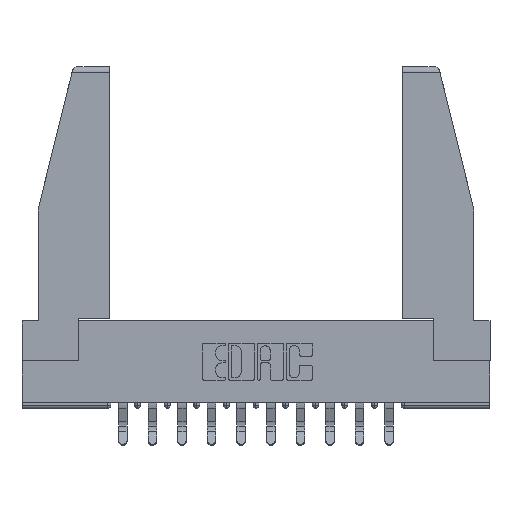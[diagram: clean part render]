
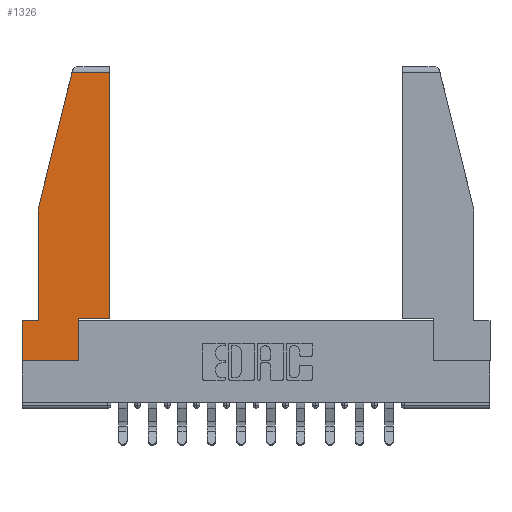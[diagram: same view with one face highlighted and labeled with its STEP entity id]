
A CAD part, top view. The second image highlights one B-rep face of the part: STEP entity #1326.
In plain terms, the highlighted planar face has unit normal (0, 0, 1).
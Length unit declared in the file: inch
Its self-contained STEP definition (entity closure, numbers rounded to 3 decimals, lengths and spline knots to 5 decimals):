
#252 = VERTEX_POINT ( 'NONE', #12248 ) ;
#356 = DIRECTION ( 'NONE',  ( 0., -1., 0. ) ) ;
#734 = VECTOR ( 'NONE', #16196, 39.37008 ) ;
#753 = EDGE_CURVE ( 'NONE', #14464, #252, #7016, .T. ) ;
#931 = LINE ( 'NONE', #16263, #734 ) ;
#1299 = DIRECTION ( 'NONE',  ( -1., 0., 0. ) ) ;
#1326 = ADVANCED_FACE ( 'NONE', ( #11200 ), #15914, .T. ) ;
#1522 = LINE ( 'NONE', #8565, #10340 ) ;
#1701 = ORIENTED_EDGE ( 'NONE', *, *, #16197, .T. ) ;
#1985 = CARTESIAN_POINT ( 'NONE',  ( 0., 0.21, 0. ) ) ;
#2425 = DIRECTION ( 'NONE',  ( 0., -1., 0. ) ) ;
#3075 = EDGE_CURVE ( 'NONE', #12537, #5365, #11976, .T. ) ;
#3438 = VECTOR ( 'NONE', #1299, 39.37008 ) ;
#3572 = AXIS2_PLACEMENT_3D ( 'NONE', #12133, #5305, #13537 ) ;
#3636 = ORIENTED_EDGE ( 'NONE', *, *, #753, .T. ) ;
#3857 = CARTESIAN_POINT ( 'NONE',  ( 0., 1.52, 0. ) ) ;
#3923 = LINE ( 'NONE', #7523, #7714 ) ;
#4190 = VECTOR ( 'NONE', #8435, 39.37008 ) ;
#4196 = DIRECTION ( 'NONE',  ( -0.239, -0.971, 0. ) ) ;
#4378 = CARTESIAN_POINT ( 'NONE',  ( 0., 0., 0. ) ) ;
#4579 = EDGE_CURVE ( 'NONE', #252, #11981, #16111, .T. ) ;
#4947 = EDGE_CURVE ( 'NONE', #11981, #9385, #11437, .T. ) ;
#5299 = VECTOR ( 'NONE', #14900, 39.37008 ) ;
#5305 = DIRECTION ( 'NONE',  ( 0., 0., 1. ) ) ;
#5344 = CARTESIAN_POINT ( 'NONE',  ( 0.297, 0., 0. ) ) ;
#5365 = VERTEX_POINT ( 'NONE', #10598 ) ;
#5548 = ORIENTED_EDGE ( 'NONE', *, *, #4947, .T. ) ;
#5598 = CARTESIAN_POINT ( 'NONE',  ( 0.297, 0.223, 0. ) ) ;
#5973 = VECTOR ( 'NONE', #4196, 39.37008 ) ;
#6244 = VERTEX_POINT ( 'NONE', #1985 ) ;
#6564 = CARTESIAN_POINT ( 'NONE',  ( 0.297, 0.223, 0. ) ) ;
#6566 = LINE ( 'NONE', #6564, #5299 ) ;
#6943 = ORIENTED_EDGE ( 'NONE', *, *, #4579, .T. ) ;
#7007 = ORIENTED_EDGE ( 'NONE', *, *, #16994, .T. ) ;
#7016 = LINE ( 'NONE', #3857, #3438 ) ;
#7520 = CARTESIAN_POINT ( 'NONE',  ( 0., 0., 0. ) ) ;
#7523 = CARTESIAN_POINT ( 'NONE',  ( 0.461, 0.223, 0. ) ) ;
#7702 = EDGE_CURVE ( 'NONE', #5365, #8466, #13246, .T. ) ;
#7714 = VECTOR ( 'NONE', #15516, 39.37008 ) ;
#8331 = CARTESIAN_POINT ( 'NONE',  ( 0.086, 0.21, 0. ) ) ;
#8435 = DIRECTION ( 'NONE',  ( 1., 0., 0. ) ) ;
#8466 = VERTEX_POINT ( 'NONE', #5598 ) ;
#8565 = CARTESIAN_POINT ( 'NONE',  ( 0., 0.21, 0. ) ) ;
#9385 = VERTEX_POINT ( 'NONE', #8331 ) ;
#9817 = EDGE_CURVE ( 'NONE', #14303, #14464, #3923, .T. ) ;
#10340 = VECTOR ( 'NONE', #356, 39.37008 ) ;
#10598 = CARTESIAN_POINT ( 'NONE',  ( 0.297, 0., 0. ) ) ;
#11030 = CARTESIAN_POINT ( 'NONE',  ( 0.461, 0.223, 0. ) ) ;
#11200 = FACE_OUTER_BOUND ( 'NONE', #13349, .T. ) ;
#11437 = LINE ( 'NONE', #17368, #16507 ) ;
#11976 = LINE ( 'NONE', #4378, #4190 ) ;
#11981 = VERTEX_POINT ( 'NONE', #14534 ) ;
#12133 = CARTESIAN_POINT ( 'NONE',  ( 0., 0., 0. ) ) ;
#12248 = CARTESIAN_POINT ( 'NONE',  ( 0.2636, 1.52, 0. ) ) ;
#12537 = VERTEX_POINT ( 'NONE', #7520 ) ;
#13170 = CARTESIAN_POINT ( 'NONE',  ( 0.461, 1.52, 0. ) ) ;
#13246 = LINE ( 'NONE', #5344, #17272 ) ;
#13349 = EDGE_LOOP ( 'NONE', ( #15074, #3636, #6943, #5548, #1701, #7007, #16405, #15811, #16738 ) ) ;
#13537 = DIRECTION ( 'NONE',  ( 1., 0., 0. ) ) ;
#13775 = CARTESIAN_POINT ( 'NONE',  ( 0.271, 1.55, 0. ) ) ;
#14303 = VERTEX_POINT ( 'NONE', #11030 ) ;
#14464 = VERTEX_POINT ( 'NONE', #13170 ) ;
#14534 = CARTESIAN_POINT ( 'NONE',  ( 0.086, 0.8, 0. ) ) ;
#14743 = DIRECTION ( 'NONE',  ( 0., 1., 0. ) ) ;
#14900 = DIRECTION ( 'NONE',  ( 1., 0., 0. ) ) ;
#15074 = ORIENTED_EDGE ( 'NONE', *, *, #9817, .T. ) ;
#15516 = DIRECTION ( 'NONE',  ( 0., 1., 0. ) ) ;
#15811 = ORIENTED_EDGE ( 'NONE', *, *, #7702, .T. ) ;
#15914 = PLANE ( 'NONE',  #3572 ) ;
#16111 = LINE ( 'NONE', #13775, #5973 ) ;
#16196 = DIRECTION ( 'NONE',  ( -1., 0., 0. ) ) ;
#16197 = EDGE_CURVE ( 'NONE', #9385, #6244, #931, .T. ) ;
#16263 = CARTESIAN_POINT ( 'NONE',  ( 0., 0.21, 0. ) ) ;
#16405 = ORIENTED_EDGE ( 'NONE', *, *, #3075, .T. ) ;
#16507 = VECTOR ( 'NONE', #2425, 39.37008 ) ;
#16738 = ORIENTED_EDGE ( 'NONE', *, *, #16887, .T. ) ;
#16887 = EDGE_CURVE ( 'NONE', #8466, #14303, #6566, .T. ) ;
#16994 = EDGE_CURVE ( 'NONE', #6244, #12537, #1522, .T. ) ;
#17272 = VECTOR ( 'NONE', #14743, 39.37008 ) ;
#17368 = CARTESIAN_POINT ( 'NONE',  ( 0.086, 0.8, 0. ) ) ;
